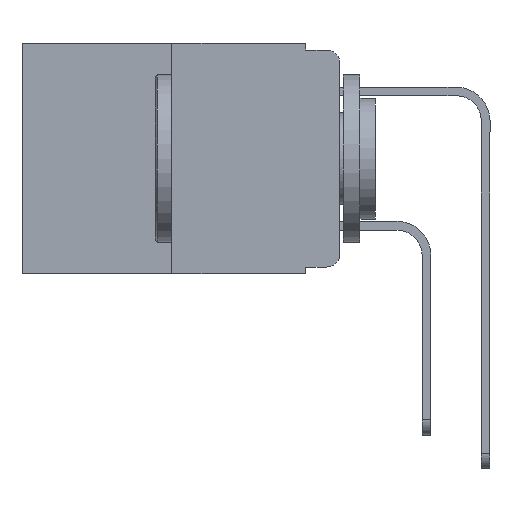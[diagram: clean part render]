
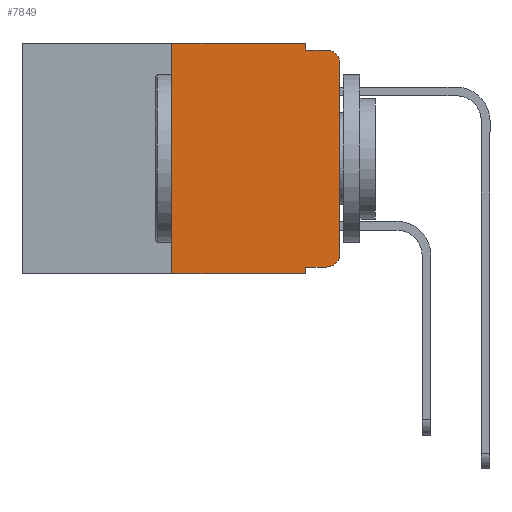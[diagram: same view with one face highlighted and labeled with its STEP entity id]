
A CAD part, left-side view. The second image highlights one B-rep face of the part: STEP entity #7849.
In plain terms, the highlighted planar face has unit normal (-1, 0, 0).
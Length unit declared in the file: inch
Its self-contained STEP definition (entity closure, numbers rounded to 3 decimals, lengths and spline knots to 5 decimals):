
#234 = EDGE_CURVE ( 'NONE', #6112, #4412, #7033, .T. ) ;
#312 = VECTOR ( 'NONE', #10974, 39.37008 ) ;
#489 = DIRECTION ( 'NONE',  ( 0., 0., -1. ) ) ;
#520 = ORIENTED_EDGE ( 'NONE', *, *, #1672, .T. ) ;
#695 = PLANE ( 'NONE',  #6059 ) ;
#707 = AXIS2_PLACEMENT_3D ( 'NONE', #12720, #5252, #12646 ) ;
#1363 = ORIENTED_EDGE ( 'NONE', *, *, #4802, .F. ) ;
#1445 = CARTESIAN_POINT ( 'NONE',  ( 0., 0.02, -0.333 ) ) ;
#1672 = EDGE_CURVE ( 'NONE', #6112, #7023, #11538, .T. ) ;
#1695 = CARTESIAN_POINT ( 'NONE',  ( 0., 0.473, -0.343 ) ) ;
#2027 = ORIENTED_EDGE ( 'NONE', *, *, #8685, .F. ) ;
#2088 = CARTESIAN_POINT ( 'NONE',  ( 0., 0.25, -0.343 ) ) ;
#2300 = DIRECTION ( 'NONE',  ( 0., 0., -1. ) ) ;
#2313 = DIRECTION ( 'NONE',  ( -1., 0., 0. ) ) ;
#2323 = CARTESIAN_POINT ( 'NONE',  ( 0., 0.02, -0.03 ) ) ;
#2401 = DIRECTION ( 'NONE',  ( 0., -1., 0. ) ) ;
#2633 = EDGE_CURVE ( 'NONE', #3800, #9887, #5643, .T. ) ;
#2673 = VERTEX_POINT ( 'NONE', #2088 ) ;
#2818 = CARTESIAN_POINT ( 'NONE',  ( 0., 0.02, -0.01 ) ) ;
#2857 = ORIENTED_EDGE ( 'NONE', *, *, #9304, .T. ) ;
#3203 = ORIENTED_EDGE ( 'NONE', *, *, #2633, .T. ) ;
#3531 = VECTOR ( 'NONE', #9645, 39.37008 ) ;
#3559 = CARTESIAN_POINT ( 'NONE',  ( 0., 0.051, -0.333 ) ) ;
#3763 = VERTEX_POINT ( 'NONE', #12851 ) ;
#3797 = CARTESIAN_POINT ( 'NONE',  ( 0., 0.051, 0. ) ) ;
#3800 = VERTEX_POINT ( 'NONE', #12178 ) ;
#3826 = EDGE_CURVE ( 'NONE', #7023, #3763, #5675, .T. ) ;
#3911 = DIRECTION ( 'NONE',  ( 0., 0., 1. ) ) ;
#3933 = DIRECTION ( 'NONE',  ( 1., 0., 0. ) ) ;
#4323 = VECTOR ( 'NONE', #11982, 39.37008 ) ;
#4350 = EDGE_LOOP ( 'NONE', ( #2857, #3203, #9489, #1363, #2027, #13165, #8341, #8660, #520, #6550 ) ) ;
#4371 = EDGE_CURVE ( 'NONE', #2673, #4412, #9591, .T. ) ;
#4412 = VERTEX_POINT ( 'NONE', #11247 ) ;
#4655 = LINE ( 'NONE', #13202, #4323 ) ;
#4726 = VERTEX_POINT ( 'NONE', #3797 ) ;
#4802 = EDGE_CURVE ( 'NONE', #4726, #9758, #10091, .T. ) ;
#5064 = EDGE_CURVE ( 'NONE', #9758, #9887, #4655, .T. ) ;
#5136 = VERTEX_POINT ( 'NONE', #9159 ) ;
#5244 = VECTOR ( 'NONE', #3911, 39.37008 ) ;
#5252 = DIRECTION ( 'NONE',  ( -1., 0., 0. ) ) ;
#5371 = LINE ( 'NONE', #5980, #9496 ) ;
#5529 = VECTOR ( 'NONE', #8262, 39.37008 ) ;
#5643 = CIRCLE ( 'NONE', #5644, 0.02 ) ;
#5644 = AXIS2_PLACEMENT_3D ( 'NONE', #2323, #2313, #2300 ) ;
#5675 = CIRCLE ( 'NONE', #707, 0.02 ) ;
#5980 = CARTESIAN_POINT ( 'NONE',  ( 0., 0.473, 0. ) ) ;
#6059 = AXIS2_PLACEMENT_3D ( 'NONE', #7103, #3933, #11275 ) ;
#6112 = VERTEX_POINT ( 'NONE', #3559 ) ;
#6193 = LINE ( 'NONE', #7220, #5529 ) ;
#6550 = ORIENTED_EDGE ( 'NONE', *, *, #3826, .T. ) ;
#6811 = VECTOR ( 'NONE', #13014, 39.37008 ) ;
#7023 = VERTEX_POINT ( 'NONE', #1445 ) ;
#7033 = LINE ( 'NONE', #9527, #3531 ) ;
#7103 = CARTESIAN_POINT ( 'NONE',  ( 0., 0.473, 0. ) ) ;
#7220 = CARTESIAN_POINT ( 'NONE',  ( 0., 0., 0. ) ) ;
#7319 = VECTOR ( 'NONE', #489, 39.37008 ) ;
#7849 = ADVANCED_FACE ( 'NONE', ( #12390 ), #695, .F. ) ;
#8059 = LINE ( 'NONE', #13257, #5244 ) ;
#8262 = DIRECTION ( 'NONE',  ( 0., 0., 1. ) ) ;
#8341 = ORIENTED_EDGE ( 'NONE', *, *, #4371, .T. ) ;
#8365 = CARTESIAN_POINT ( 'NONE',  ( 0., 0.051, -0.333 ) ) ;
#8660 = ORIENTED_EDGE ( 'NONE', *, *, #234, .F. ) ;
#8685 = EDGE_CURVE ( 'NONE', #5136, #4726, #5371, .T. ) ;
#8931 = CARTESIAN_POINT ( 'NONE',  ( 0., 0.051, 0. ) ) ;
#9159 = CARTESIAN_POINT ( 'NONE',  ( 0., 0.25, 0. ) ) ;
#9304 = EDGE_CURVE ( 'NONE', #3763, #3800, #6193, .T. ) ;
#9489 = ORIENTED_EDGE ( 'NONE', *, *, #5064, .F. ) ;
#9496 = VECTOR ( 'NONE', #2401, 39.37008 ) ;
#9527 = CARTESIAN_POINT ( 'NONE',  ( 0., 0.051, 0. ) ) ;
#9591 = LINE ( 'NONE', #1695, #6811 ) ;
#9645 = DIRECTION ( 'NONE',  ( 0., 0., -1. ) ) ;
#9758 = VERTEX_POINT ( 'NONE', #10038 ) ;
#9887 = VERTEX_POINT ( 'NONE', #2818 ) ;
#10038 = CARTESIAN_POINT ( 'NONE',  ( 0., 0.051, -0.01 ) ) ;
#10091 = LINE ( 'NONE', #8931, #7319 ) ;
#10974 = DIRECTION ( 'NONE',  ( 0., -1., 0. ) ) ;
#11120 = EDGE_CURVE ( 'NONE', #2673, #5136, #8059, .T. ) ;
#11247 = CARTESIAN_POINT ( 'NONE',  ( 0., 0.051, -0.343 ) ) ;
#11275 = DIRECTION ( 'NONE',  ( 0., 0., -1. ) ) ;
#11538 = LINE ( 'NONE', #8365, #312 ) ;
#11982 = DIRECTION ( 'NONE',  ( 0., -1., 0. ) ) ;
#12178 = CARTESIAN_POINT ( 'NONE',  ( 0., 0., -0.03 ) ) ;
#12390 = FACE_OUTER_BOUND ( 'NONE', #4350, .T. ) ;
#12646 = DIRECTION ( 'NONE',  ( 0., 0., -1. ) ) ;
#12720 = CARTESIAN_POINT ( 'NONE',  ( 0., 0.02, -0.313 ) ) ;
#12851 = CARTESIAN_POINT ( 'NONE',  ( 0., 0., -0.313 ) ) ;
#13014 = DIRECTION ( 'NONE',  ( 0., -1., 0. ) ) ;
#13165 = ORIENTED_EDGE ( 'NONE', *, *, #11120, .F. ) ;
#13202 = CARTESIAN_POINT ( 'NONE',  ( 0., 0.051, -0.01 ) ) ;
#13257 = CARTESIAN_POINT ( 'NONE',  ( 0., 0.25, 0. ) ) ;
